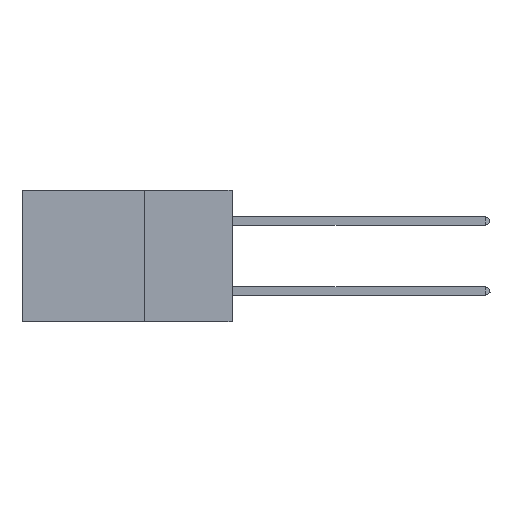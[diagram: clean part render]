
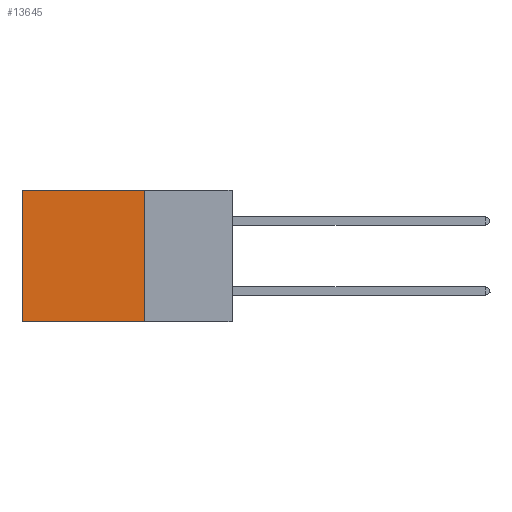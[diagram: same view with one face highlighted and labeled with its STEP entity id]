
A CAD part, left-side view. The second image highlights one B-rep face of the part: STEP entity #13645.
In plain terms, the highlighted planar face has unit normal (-1, 0, 0).
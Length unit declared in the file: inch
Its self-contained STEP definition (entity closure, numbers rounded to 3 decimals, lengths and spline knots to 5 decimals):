
#1051 = CARTESIAN_POINT ( 'NONE',  ( 0.2875, 0.25, -0.375 ) ) ;
#1194 = ORIENTED_EDGE ( 'NONE', *, *, #10792, .F. ) ;
#2920 = EDGE_CURVE ( 'NONE', #13572, #16000, #8609, .T. ) ;
#3242 = VERTEX_POINT ( 'NONE', #16467 ) ;
#3432 = ORIENTED_EDGE ( 'NONE', *, *, #2920, .T. ) ;
#3959 = VERTEX_POINT ( 'NONE', #21694 ) ;
#4775 = VECTOR ( 'NONE', #5162, 39.37008 ) ;
#5162 = DIRECTION ( 'NONE',  ( 0., 0., -1. ) ) ;
#5273 = CARTESIAN_POINT ( 'NONE',  ( 0.2875, 0.25, -0.375 ) ) ;
#5551 = EDGE_LOOP ( 'NONE', ( #10847, #12575, #1194, #3432 ) ) ;
#5820 = LINE ( 'NONE', #16672, #4775 ) ;
#6734 = DIRECTION ( 'NONE',  ( 0., 0., -1. ) ) ;
#7018 = DIRECTION ( 'NONE',  ( 0., 0., -1. ) ) ;
#7365 = CARTESIAN_POINT ( 'NONE',  ( 0.2875, 0.25, 0. ) ) ;
#8609 = LINE ( 'NONE', #7365, #19643 ) ;
#8893 = CARTESIAN_POINT ( 'NONE',  ( 0.2875, 0.25, 0. ) ) ;
#9380 = DIRECTION ( 'NONE',  ( 0., 1., 0. ) ) ;
#9593 = FACE_OUTER_BOUND ( 'NONE', #5551, .T. ) ;
#10535 = LINE ( 'NONE', #1051, #18910 ) ;
#10792 = EDGE_CURVE ( 'NONE', #13572, #3959, #14763, .T. ) ;
#10847 = ORIENTED_EDGE ( 'NONE', *, *, #15195, .T. ) ;
#12037 = EDGE_CURVE ( 'NONE', #3959, #3242, #10535, .T. ) ;
#12141 = DIRECTION ( 'NONE',  ( 1., 0., 0. ) ) ;
#12575 = ORIENTED_EDGE ( 'NONE', *, *, #12037, .F. ) ;
#13572 = VERTEX_POINT ( 'NONE', #8893 ) ;
#13645 = ADVANCED_FACE ( 'NONE', ( #9593 ), #18990, .F. ) ;
#14063 = DIRECTION ( 'NONE',  ( 0., 1., 0. ) ) ;
#14763 = LINE ( 'NONE', #5273, #17358 ) ;
#15195 = EDGE_CURVE ( 'NONE', #16000, #3242, #5820, .T. ) ;
#16000 = VERTEX_POINT ( 'NONE', #17836 ) ;
#16467 = CARTESIAN_POINT ( 'NONE',  ( 0.2875, 0.6, -0.375 ) ) ;
#16672 = CARTESIAN_POINT ( 'NONE',  ( 0.2875, 0.6, -0.375 ) ) ;
#17216 = CARTESIAN_POINT ( 'NONE',  ( 0.2875, 0.25, -0.375 ) ) ;
#17358 = VECTOR ( 'NONE', #6734, 39.37008 ) ;
#17836 = CARTESIAN_POINT ( 'NONE',  ( 0.2875, 0.6, 0. ) ) ;
#18593 = AXIS2_PLACEMENT_3D ( 'NONE', #17216, #12141, #7018 ) ;
#18910 = VECTOR ( 'NONE', #9380, 39.37008 ) ;
#18990 = PLANE ( 'NONE',  #18593 ) ;
#19643 = VECTOR ( 'NONE', #14063, 39.37008 ) ;
#21694 = CARTESIAN_POINT ( 'NONE',  ( 0.2875, 0.25, -0.375 ) ) ;
